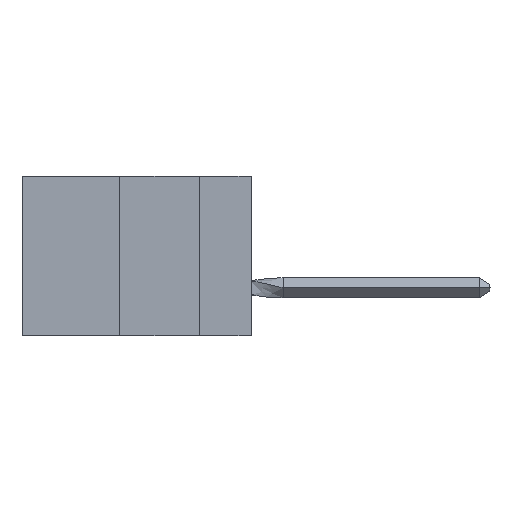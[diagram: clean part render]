
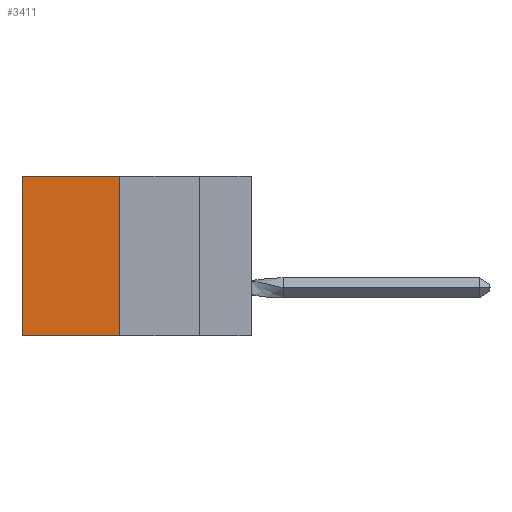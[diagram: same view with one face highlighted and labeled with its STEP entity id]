
A CAD part, left-side view. The second image highlights one B-rep face of the part: STEP entity #3411.
In plain terms, the highlighted planar face has unit normal (-1, 0, 0).
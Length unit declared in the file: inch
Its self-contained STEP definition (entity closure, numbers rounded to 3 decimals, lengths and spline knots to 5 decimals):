
#26 = VERTEX_POINT ( 'NONE', #9685 ) ;
#422 = DIRECTION ( 'NONE',  ( 1., 0., 0. ) ) ;
#589 = LINE ( 'NONE', #4005, #13197 ) ;
#1255 = CARTESIAN_POINT ( 'NONE',  ( 0.305, 0.413, -0.5 ) ) ;
#3196 = VERTEX_POINT ( 'NONE', #10716 ) ;
#3411 = ADVANCED_FACE ( 'NONE', ( #10063 ), #7021, .F. ) ;
#3483 = EDGE_CURVE ( 'NONE', #21256, #26, #15200, .T. ) ;
#4005 = CARTESIAN_POINT ( 'NONE',  ( 0.305, 0.413, 0. ) ) ;
#4102 = ORIENTED_EDGE ( 'NONE', *, *, #5795, .F. ) ;
#5101 = VECTOR ( 'NONE', #7791, 39.37008 ) ;
#5795 = EDGE_CURVE ( 'NONE', #26, #3196, #13857, .T. ) ;
#6337 = ORIENTED_EDGE ( 'NONE', *, *, #3483, .F. ) ;
#6828 = ORIENTED_EDGE ( 'NONE', *, *, #18259, .T. ) ;
#7021 = PLANE ( 'NONE',  #8494 ) ;
#7358 = DIRECTION ( 'NONE',  ( 0., 0., -1. ) ) ;
#7791 = DIRECTION ( 'NONE',  ( 0., 1., 0. ) ) ;
#8494 = AXIS2_PLACEMENT_3D ( 'NONE', #15095, #422, #10404 ) ;
#8663 = LINE ( 'NONE', #10587, #9420 ) ;
#8901 = CARTESIAN_POINT ( 'NONE',  ( 0.305, 0.72, 0. ) ) ;
#9420 = VECTOR ( 'NONE', #7358, 39.37008 ) ;
#9685 = CARTESIAN_POINT ( 'NONE',  ( 0.305, 0.413, -0.5 ) ) ;
#10063 = FACE_OUTER_BOUND ( 'NONE', #17868, .T. ) ;
#10404 = DIRECTION ( 'NONE',  ( 0., 0., -1. ) ) ;
#10587 = CARTESIAN_POINT ( 'NONE',  ( 0.305, 0.72, -0.5 ) ) ;
#10716 = CARTESIAN_POINT ( 'NONE',  ( 0.305, 0.72, -0.5 ) ) ;
#12069 = DIRECTION ( 'NONE',  ( 0., 0., -1. ) ) ;
#12826 = EDGE_CURVE ( 'NONE', #21016, #3196, #8663, .T. ) ;
#13197 = VECTOR ( 'NONE', #20702, 39.37008 ) ;
#13857 = LINE ( 'NONE', #1255, #5101 ) ;
#15095 = CARTESIAN_POINT ( 'NONE',  ( 0.305, 0.413, -0.5 ) ) ;
#15200 = LINE ( 'NONE', #16693, #17291 ) ;
#16693 = CARTESIAN_POINT ( 'NONE',  ( 0.305, 0.413, -0.5 ) ) ;
#17291 = VECTOR ( 'NONE', #12069, 39.37008 ) ;
#17455 = CARTESIAN_POINT ( 'NONE',  ( 0.305, 0.413, 0. ) ) ;
#17868 = EDGE_LOOP ( 'NONE', ( #20587, #4102, #6337, #6828 ) ) ;
#18259 = EDGE_CURVE ( 'NONE', #21256, #21016, #589, .T. ) ;
#20587 = ORIENTED_EDGE ( 'NONE', *, *, #12826, .T. ) ;
#20702 = DIRECTION ( 'NONE',  ( 0., 1., 0. ) ) ;
#21016 = VERTEX_POINT ( 'NONE', #8901 ) ;
#21256 = VERTEX_POINT ( 'NONE', #17455 ) ;
